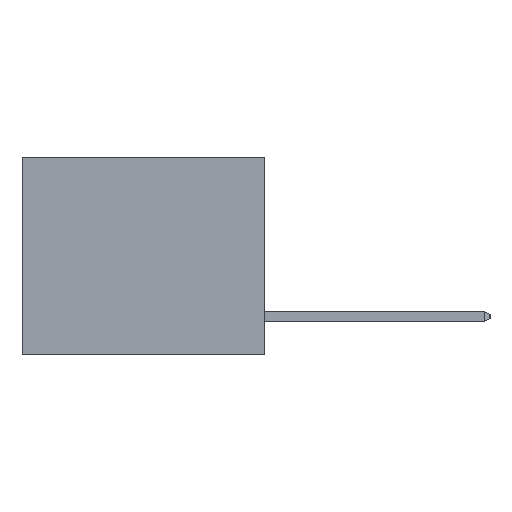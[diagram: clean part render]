
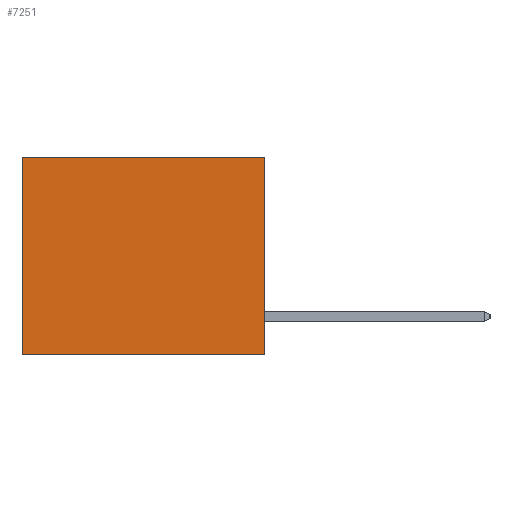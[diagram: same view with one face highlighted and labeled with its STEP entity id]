
A CAD part, left-side view. The second image highlights one B-rep face of the part: STEP entity #7251.
In plain terms, the highlighted planar face has unit normal (-1, 0, 0).
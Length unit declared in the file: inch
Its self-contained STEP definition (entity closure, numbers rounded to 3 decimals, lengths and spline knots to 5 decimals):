
#248 = CARTESIAN_POINT ( 'NONE',  ( 0.3165, 0., 0. ) ) ;
#447 = ORIENTED_EDGE ( 'NONE', *, *, #20947, .T. ) ;
#819 = VERTEX_POINT ( 'NONE', #3144 ) ;
#1700 = CARTESIAN_POINT ( 'NONE',  ( 0.3165, 0., 0. ) ) ;
#2650 = LINE ( 'NONE', #9970, #21714 ) ;
#2879 = DIRECTION ( 'NONE',  ( 1., 0., 0. ) ) ;
#3144 = CARTESIAN_POINT ( 'NONE',  ( 0.3165, 0., -0.49 ) ) ;
#3770 = ORIENTED_EDGE ( 'NONE', *, *, #23693, .T. ) ;
#4569 = VERTEX_POINT ( 'NONE', #8619 ) ;
#4721 = VECTOR ( 'NONE', #18251, 39.37008 ) ;
#5348 = CARTESIAN_POINT ( 'NONE',  ( 0.3165, 0., -0.49 ) ) ;
#6184 = EDGE_CURVE ( 'NONE', #819, #7382, #18382, .T. ) ;
#6609 = PLANE ( 'NONE',  #13408 ) ;
#7251 = ADVANCED_FACE ( 'NONE', ( #8805 ), #6609, .F. ) ;
#7379 = EDGE_CURVE ( 'NONE', #19725, #819, #13461, .T. ) ;
#7382 = VERTEX_POINT ( 'NONE', #18329 ) ;
#8619 = CARTESIAN_POINT ( 'NONE',  ( 0.3165, 0.6, 0. ) ) ;
#8805 = FACE_OUTER_BOUND ( 'NONE', #20370, .T. ) ;
#9970 = CARTESIAN_POINT ( 'NONE',  ( 0.3165, 0.6, -0.49 ) ) ;
#12708 = CARTESIAN_POINT ( 'NONE',  ( 0.3165, 0., -0.49 ) ) ;
#13408 = AXIS2_PLACEMENT_3D ( 'NONE', #21290, #2879, #15547 ) ;
#13461 = LINE ( 'NONE', #12708, #4721 ) ;
#14373 = VECTOR ( 'NONE', #20380, 39.37008 ) ;
#15547 = DIRECTION ( 'NONE',  ( 0., 0., -1. ) ) ;
#15836 = VECTOR ( 'NONE', #16772, 39.37008 ) ;
#16772 = DIRECTION ( 'NONE',  ( 0., 1., 0. ) ) ;
#17591 = LINE ( 'NONE', #1700, #15836 ) ;
#18251 = DIRECTION ( 'NONE',  ( 0., 0., -1. ) ) ;
#18329 = CARTESIAN_POINT ( 'NONE',  ( 0.3165, 0.6, -0.49 ) ) ;
#18382 = LINE ( 'NONE', #5348, #14373 ) ;
#19725 = VERTEX_POINT ( 'NONE', #248 ) ;
#20370 = EDGE_LOOP ( 'NONE', ( #447, #22169, #21442, #3770 ) ) ;
#20380 = DIRECTION ( 'NONE',  ( 0., 1., 0. ) ) ;
#20947 = EDGE_CURVE ( 'NONE', #4569, #7382, #2650, .T. ) ;
#21290 = CARTESIAN_POINT ( 'NONE',  ( 0.3165, 0., -0.49 ) ) ;
#21442 = ORIENTED_EDGE ( 'NONE', *, *, #7379, .F. ) ;
#21714 = VECTOR ( 'NONE', #22876, 39.37008 ) ;
#22169 = ORIENTED_EDGE ( 'NONE', *, *, #6184, .F. ) ;
#22876 = DIRECTION ( 'NONE',  ( 0., 0., -1. ) ) ;
#23693 = EDGE_CURVE ( 'NONE', #19725, #4569, #17591, .T. ) ;
